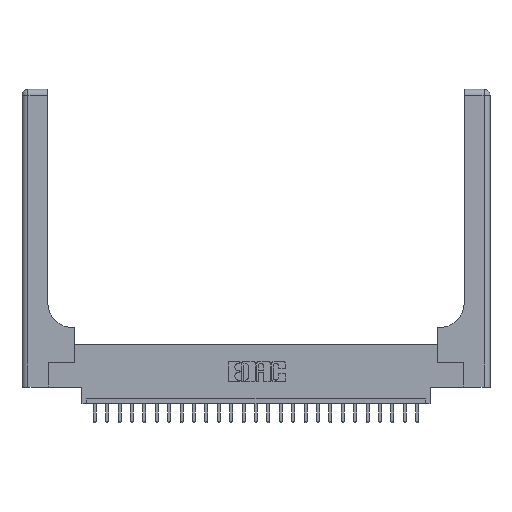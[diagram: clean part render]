
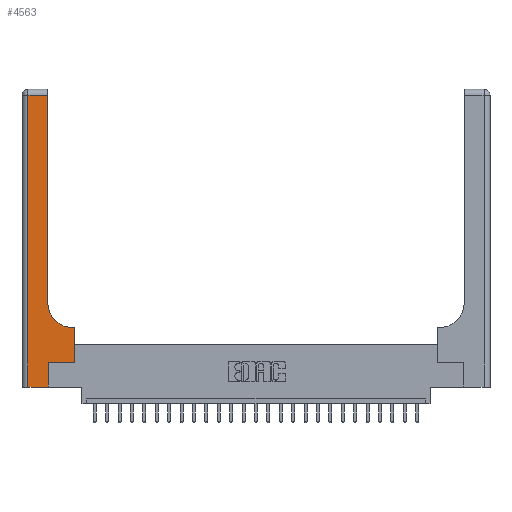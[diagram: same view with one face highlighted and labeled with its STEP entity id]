
A CAD part, top view. The second image highlights one B-rep face of the part: STEP entity #4563.
In plain terms, the highlighted planar face has unit normal (0, 0, 1).
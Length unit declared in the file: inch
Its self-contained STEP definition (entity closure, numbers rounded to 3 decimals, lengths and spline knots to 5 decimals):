
#114 = CARTESIAN_POINT ( 'NONE',  ( 0.265, 0., 0.37 ) ) ;
#243 = LINE ( 'NONE', #114, #3740 ) ;
#258 = LINE ( 'NONE', #17600, #4256 ) ;
#623 = DIRECTION ( 'NONE',  ( 0., -1., 0. ) ) ;
#652 = ORIENTED_EDGE ( 'NONE', *, *, #4280, .T. ) ;
#727 = DIRECTION ( 'NONE',  ( 1., 0., 0. ) ) ;
#975 = LINE ( 'NONE', #17807, #5860 ) ;
#1324 = VECTOR ( 'NONE', #623, 39.37008 ) ;
#1551 = CARTESIAN_POINT ( 'NONE',  ( 0.26, 3., 0.37 ) ) ;
#1632 = CARTESIAN_POINT ( 'NONE',  ( 0.265, 0., 0.37 ) ) ;
#1713 = CARTESIAN_POINT ( 'NONE',  ( 0.265, 0.25, 0.37 ) ) ;
#1993 = CARTESIAN_POINT ( 'NONE',  ( 0.51, 0.6, 0.37 ) ) ;
#2306 = EDGE_CURVE ( 'NONE', #11004, #17141, #6520, .T. ) ;
#2624 = DIRECTION ( 'NONE',  ( 1., 0., 0. ) ) ;
#2628 = ORIENTED_EDGE ( 'NONE', *, *, #16729, .T. ) ;
#3141 = DIRECTION ( 'NONE',  ( 0., 1., 0. ) ) ;
#3635 = VERTEX_POINT ( 'NONE', #1632 ) ;
#3716 = VERTEX_POINT ( 'NONE', #24455 ) ;
#3740 = VECTOR ( 'NONE', #7738, 39.37008 ) ;
#3834 = LINE ( 'NONE', #13707, #21776 ) ;
#4053 = CARTESIAN_POINT ( 'NONE',  ( 0.51, 0.85, 0.37 ) ) ;
#4256 = VECTOR ( 'NONE', #2624, 39.37008 ) ;
#4280 = EDGE_CURVE ( 'NONE', #17141, #16613, #3834, .T. ) ;
#4563 = ADVANCED_FACE ( 'NONE', ( #12939 ), #20659, .F. ) ;
#5561 = CARTESIAN_POINT ( 'NONE',  ( 0., 3., 0.37 ) ) ;
#5860 = VECTOR ( 'NONE', #727, 39.37008 ) ;
#5947 = CARTESIAN_POINT ( 'NONE',  ( 0.528, 0.25, 0.37 ) ) ;
#6458 = ORIENTED_EDGE ( 'NONE', *, *, #2306, .T. ) ;
#6520 = LINE ( 'NONE', #21973, #13007 ) ;
#6560 = VERTEX_POINT ( 'NONE', #17849 ) ;
#7425 = LINE ( 'NONE', #1551, #21885 ) ;
#7738 = DIRECTION ( 'NONE',  ( 0., 1., 0. ) ) ;
#7862 = AXIS2_PLACEMENT_3D ( 'NONE', #4053, #13418, #22771 ) ;
#7987 = CARTESIAN_POINT ( 'NONE',  ( 0.06, 3., 0.37 ) ) ;
#8272 = CARTESIAN_POINT ( 'NONE',  ( 0.26, 2.94, 0.37 ) ) ;
#8727 = CARTESIAN_POINT ( 'NONE',  ( 0.528, 0.6, 0.37 ) ) ;
#9326 = CARTESIAN_POINT ( 'NONE',  ( 0., 2.94, 0.37 ) ) ;
#9439 = DIRECTION ( 'NONE',  ( -1., 0., 0. ) ) ;
#9855 = LINE ( 'NONE', #7987, #1324 ) ;
#10741 = EDGE_CURVE ( 'NONE', #23169, #3716, #9855, .T. ) ;
#11004 = VERTEX_POINT ( 'NONE', #5947 ) ;
#11056 = ORIENTED_EDGE ( 'NONE', *, *, #11921, .T. ) ;
#11155 = EDGE_LOOP ( 'NONE', ( #13428, #14138, #11695, #2628, #11056, #18353, #6458, #652, #14163 ) ) ;
#11446 = LINE ( 'NONE', #9326, #16653 ) ;
#11695 = ORIENTED_EDGE ( 'NONE', *, *, #10741, .T. ) ;
#11921 = EDGE_CURVE ( 'NONE', #3635, #12156, #243, .T. ) ;
#12156 = VERTEX_POINT ( 'NONE', #1713 ) ;
#12939 = FACE_OUTER_BOUND ( 'NONE', #11155, .T. ) ;
#13007 = VECTOR ( 'NONE', #3141, 39.37008 ) ;
#13418 = DIRECTION ( 'NONE',  ( 0., 0., -1. ) ) ;
#13428 = ORIENTED_EDGE ( 'NONE', *, *, #20154, .T. ) ;
#13707 = CARTESIAN_POINT ( 'NONE',  ( 0.26, 0.6, 0.37 ) ) ;
#14138 = ORIENTED_EDGE ( 'NONE', *, *, #18524, .T. ) ;
#14163 = ORIENTED_EDGE ( 'NONE', *, *, #17486, .T. ) ;
#15840 = AXIS2_PLACEMENT_3D ( 'NONE', #5561, #18790, #9439 ) ;
#16613 = VERTEX_POINT ( 'NONE', #1993 ) ;
#16653 = VECTOR ( 'NONE', #19038, 39.37008 ) ;
#16729 = EDGE_CURVE ( 'NONE', #3716, #3635, #258, .T. ) ;
#17141 = VERTEX_POINT ( 'NONE', #8727 ) ;
#17281 = EDGE_CURVE ( 'NONE', #12156, #11004, #975, .T. ) ;
#17318 = DIRECTION ( 'NONE',  ( -1., 0., 0. ) ) ;
#17486 = EDGE_CURVE ( 'NONE', #16613, #6560, #18610, .T. ) ;
#17600 = CARTESIAN_POINT ( 'NONE',  ( 0., 0., 0.37 ) ) ;
#17807 = CARTESIAN_POINT ( 'NONE',  ( 0.265, 0.25, 0.37 ) ) ;
#17849 = CARTESIAN_POINT ( 'NONE',  ( 0.26, 0.85, 0.37 ) ) ;
#18012 = VERTEX_POINT ( 'NONE', #8272 ) ;
#18353 = ORIENTED_EDGE ( 'NONE', *, *, #17281, .T. ) ;
#18524 = EDGE_CURVE ( 'NONE', #18012, #23169, #11446, .T. ) ;
#18610 = CIRCLE ( 'NONE', #7862, 0.25 ) ;
#18771 = DIRECTION ( 'NONE',  ( 0., 1., 0. ) ) ;
#18790 = DIRECTION ( 'NONE',  ( 0., 0., -1. ) ) ;
#19038 = DIRECTION ( 'NONE',  ( -1., 0., 0. ) ) ;
#20154 = EDGE_CURVE ( 'NONE', #6560, #18012, #7425, .T. ) ;
#20659 = PLANE ( 'NONE',  #15840 ) ;
#21398 = CARTESIAN_POINT ( 'NONE',  ( 0.06, 2.94, 0.37 ) ) ;
#21776 = VECTOR ( 'NONE', #17318, 39.37008 ) ;
#21885 = VECTOR ( 'NONE', #18771, 39.37008 ) ;
#21973 = CARTESIAN_POINT ( 'NONE',  ( 0.528, 0.25, 0.37 ) ) ;
#22771 = DIRECTION ( 'NONE',  ( 1., 0., 0. ) ) ;
#23169 = VERTEX_POINT ( 'NONE', #21398 ) ;
#24455 = CARTESIAN_POINT ( 'NONE',  ( 0.06, 0., 0.37 ) ) ;
